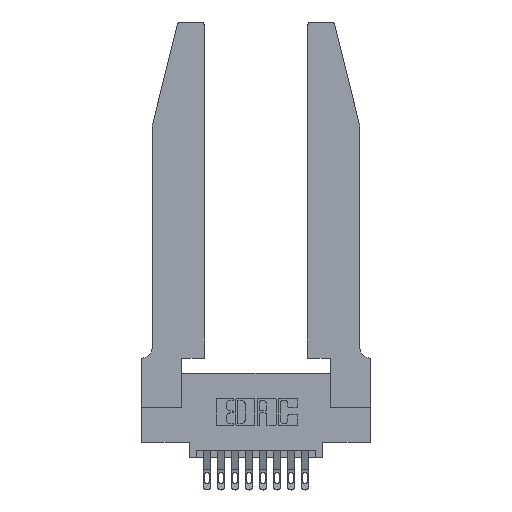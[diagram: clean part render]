
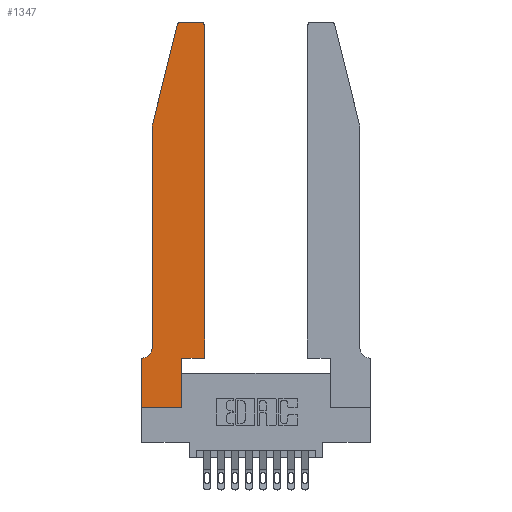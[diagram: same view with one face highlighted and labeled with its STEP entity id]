
A CAD part, top view. The second image highlights one B-rep face of the part: STEP entity #1347.
In plain terms, the highlighted planar face has unit normal (0, 0, 1).
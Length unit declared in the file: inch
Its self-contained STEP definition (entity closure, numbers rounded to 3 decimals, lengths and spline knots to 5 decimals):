
#18 = EDGE_CURVE ( 'NONE', #4099, #10882, #6035, .T. ) ;
#54 = ORIENTED_EDGE ( 'NONE', *, *, #10631, .T. ) ;
#76 = VERTEX_POINT ( 'NONE', #12419 ) ;
#234 = CARTESIAN_POINT ( 'NONE',  ( 0.0755, 0.42, 0.37 ) ) ;
#251 = VERTEX_POINT ( 'NONE', #5054 ) ;
#256 = LINE ( 'NONE', #9529, #7425 ) ;
#338 = DIRECTION ( 'NONE',  ( -1., 0., 0. ) ) ;
#1052 = ORIENTED_EDGE ( 'NONE', *, *, #12970, .T. ) ;
#1057 = DIRECTION ( 'NONE',  ( 0., 0., 1. ) ) ;
#1089 = EDGE_CURVE ( 'NONE', #10882, #13662, #3317, .T. ) ;
#1347 = ADVANCED_FACE ( 'NONE', ( #8574 ), #10369, .T. ) ;
#1619 = DIRECTION ( 'NONE',  ( 0., 0., 1. ) ) ;
#1652 = LINE ( 'NONE', #5390, #9436 ) ;
#1678 = CARTESIAN_POINT ( 'NONE',  ( 0., 0.35, 0.37 ) ) ;
#2079 = AXIS2_PLACEMENT_3D ( 'NONE', #15183, #13967, #338 ) ;
#2212 = CARTESIAN_POINT ( 'NONE',  ( 0.4505, 2.72, 0.37 ) ) ;
#2255 = VECTOR ( 'NONE', #3741, 39.37008 ) ;
#2286 = CARTESIAN_POINT ( 'NONE',  ( 0.284, 2.72, 0.37 ) ) ;
#2536 = CARTESIAN_POINT ( 'NONE',  ( 0.0755, 2., 0.37 ) ) ;
#2544 = EDGE_CURVE ( 'NONE', #5980, #9612, #14740, .T. ) ;
#2888 = CARTESIAN_POINT ( 'NONE',  ( 0.25487, 2.72718, 0.37 ) ) ;
#3143 = ORIENTED_EDGE ( 'NONE', *, *, #14225, .T. ) ;
#3239 = EDGE_CURVE ( 'NONE', #8064, #251, #9671, .T. ) ;
#3317 = CIRCLE ( 'NONE', #6085, 0.03 ) ;
#3545 = CARTESIAN_POINT ( 'NONE',  ( 0.0755, 2., 0.37 ) ) ;
#3656 = VECTOR ( 'NONE', #15004, 39.37008 ) ;
#3741 = DIRECTION ( 'NONE',  ( 0., -1., 0. ) ) ;
#4041 = AXIS2_PLACEMENT_3D ( 'NONE', #5475, #4203, #7898 ) ;
#4099 = VERTEX_POINT ( 'NONE', #14792 ) ;
#4161 = CARTESIAN_POINT ( 'NONE',  ( 0.2865, 0., 0.37 ) ) ;
#4203 = DIRECTION ( 'NONE',  ( 0., 0., 1. ) ) ;
#4337 = EDGE_CURVE ( 'NONE', #10542, #5980, #4779, .T. ) ;
#4388 = CARTESIAN_POINT ( 'NONE',  ( 0.2865, 0.35, 0.37 ) ) ;
#4777 = CARTESIAN_POINT ( 'NONE',  ( 0.0755, 0.35, 0.37 ) ) ;
#4779 = LINE ( 'NONE', #9976, #2255 ) ;
#4786 = ORIENTED_EDGE ( 'NONE', *, *, #1089, .T. ) ;
#5032 = DIRECTION ( 'NONE',  ( -0.239, -0.971, 0. ) ) ;
#5054 = CARTESIAN_POINT ( 'NONE',  ( 0.4505, 0.35, 0.37 ) ) ;
#5390 = CARTESIAN_POINT ( 'NONE',  ( 0.4505, 0.35, 0.37 ) ) ;
#5475 = CARTESIAN_POINT ( 'NONE',  ( 0.4205, 2.72, 0.37 ) ) ;
#5939 = LINE ( 'NONE', #6068, #13176 ) ;
#5980 = VERTEX_POINT ( 'NONE', #234 ) ;
#6019 = ORIENTED_EDGE ( 'NONE', *, *, #2544, .T. ) ;
#6035 = LINE ( 'NONE', #8693, #11687 ) ;
#6068 = CARTESIAN_POINT ( 'NONE',  ( 0., 0., 0.37 ) ) ;
#6085 = AXIS2_PLACEMENT_3D ( 'NONE', #2286, #1057, #10926 ) ;
#6103 = LINE ( 'NONE', #4388, #10613 ) ;
#6104 = CARTESIAN_POINT ( 'NONE',  ( 0.4505, 0.35, 0.37 ) ) ;
#6797 = ORIENTED_EDGE ( 'NONE', *, *, #3239, .T. ) ;
#6837 = AXIS2_PLACEMENT_3D ( 'NONE', #1678, #1619, #7880 ) ;
#7425 = VECTOR ( 'NONE', #14656, 39.37008 ) ;
#7534 = LINE ( 'NONE', #4777, #10651 ) ;
#7674 = EDGE_CURVE ( 'NONE', #76, #12032, #256, .T. ) ;
#7880 = DIRECTION ( 'NONE',  ( 1., 0., 0. ) ) ;
#7898 = DIRECTION ( 'NONE',  ( 1., 0., 0. ) ) ;
#8064 = VERTEX_POINT ( 'NONE', #11876 ) ;
#8346 = CARTESIAN_POINT ( 'NONE',  ( 0., 0.35, 0.37 ) ) ;
#8506 = ORIENTED_EDGE ( 'NONE', *, *, #18, .T. ) ;
#8553 = ORIENTED_EDGE ( 'NONE', *, *, #13471, .T. ) ;
#8559 = VECTOR ( 'NONE', #5032, 39.37008 ) ;
#8574 = FACE_OUTER_BOUND ( 'NONE', #9973, .T. ) ;
#8693 = CARTESIAN_POINT ( 'NONE',  ( 0.2605, 2.75, 0.37 ) ) ;
#8832 = VERTEX_POINT ( 'NONE', #8346 ) ;
#9249 = CARTESIAN_POINT ( 'NONE',  ( 0.0055, 0.35, 0.37 ) ) ;
#9436 = VECTOR ( 'NONE', #14096, 39.37008 ) ;
#9529 = CARTESIAN_POINT ( 'NONE',  ( 0., 0., 0.37 ) ) ;
#9612 = VERTEX_POINT ( 'NONE', #9249 ) ;
#9671 = LINE ( 'NONE', #6104, #3656 ) ;
#9881 = DIRECTION ( 'NONE',  ( -1., 0., 0. ) ) ;
#9917 = DIRECTION ( 'NONE',  ( -1., 0., 0. ) ) ;
#9973 = EDGE_LOOP ( 'NONE', ( #8506, #4786, #1052, #14594, #6019, #15754, #8553, #12318, #3143, #6797, #15840, #54 ) ) ;
#9976 = CARTESIAN_POINT ( 'NONE',  ( 0.0755, 2., 0.37 ) ) ;
#10082 = EDGE_CURVE ( 'NONE', #9612, #8832, #7534, .T. ) ;
#10369 = PLANE ( 'NONE',  #6837 ) ;
#10542 = VERTEX_POINT ( 'NONE', #3545 ) ;
#10613 = VECTOR ( 'NONE', #12980, 39.37008 ) ;
#10631 = EDGE_CURVE ( 'NONE', #11863, #4099, #15079, .T. ) ;
#10651 = VECTOR ( 'NONE', #9881, 39.37008 ) ;
#10882 = VERTEX_POINT ( 'NONE', #12810 ) ;
#10926 = DIRECTION ( 'NONE',  ( 1., 0., 0. ) ) ;
#11301 = DIRECTION ( 'NONE',  ( 0., -1., 0. ) ) ;
#11687 = VECTOR ( 'NONE', #9917, 39.37008 ) ;
#11863 = VERTEX_POINT ( 'NONE', #2212 ) ;
#11876 = CARTESIAN_POINT ( 'NONE',  ( 0.2865, 0.35, 0.37 ) ) ;
#12032 = VERTEX_POINT ( 'NONE', #4161 ) ;
#12318 = ORIENTED_EDGE ( 'NONE', *, *, #7674, .T. ) ;
#12419 = CARTESIAN_POINT ( 'NONE',  ( 0., 0., 0.37 ) ) ;
#12810 = CARTESIAN_POINT ( 'NONE',  ( 0.284, 2.75, 0.37 ) ) ;
#12970 = EDGE_CURVE ( 'NONE', #13662, #10542, #15106, .T. ) ;
#12980 = DIRECTION ( 'NONE',  ( 0., 1., 0. ) ) ;
#13176 = VECTOR ( 'NONE', #11301, 39.37008 ) ;
#13471 = EDGE_CURVE ( 'NONE', #8832, #76, #5939, .T. ) ;
#13662 = VERTEX_POINT ( 'NONE', #2888 ) ;
#13967 = DIRECTION ( 'NONE',  ( 0., 0., -1. ) ) ;
#14096 = DIRECTION ( 'NONE',  ( 0., 1., 0. ) ) ;
#14225 = EDGE_CURVE ( 'NONE', #12032, #8064, #6103, .T. ) ;
#14594 = ORIENTED_EDGE ( 'NONE', *, *, #4337, .T. ) ;
#14656 = DIRECTION ( 'NONE',  ( 1., 0., 0. ) ) ;
#14740 = CIRCLE ( 'NONE', #2079, 0.07 ) ;
#14792 = CARTESIAN_POINT ( 'NONE',  ( 0.4205, 2.75, 0.37 ) ) ;
#14891 = EDGE_CURVE ( 'NONE', #251, #11863, #1652, .T. ) ;
#15004 = DIRECTION ( 'NONE',  ( 1., 0., 0. ) ) ;
#15079 = CIRCLE ( 'NONE', #4041, 0.03 ) ;
#15106 = LINE ( 'NONE', #2536, #8559 ) ;
#15183 = CARTESIAN_POINT ( 'NONE',  ( 0.0055, 0.42, 0.37 ) ) ;
#15754 = ORIENTED_EDGE ( 'NONE', *, *, #10082, .T. ) ;
#15840 = ORIENTED_EDGE ( 'NONE', *, *, #14891, .T. ) ;
